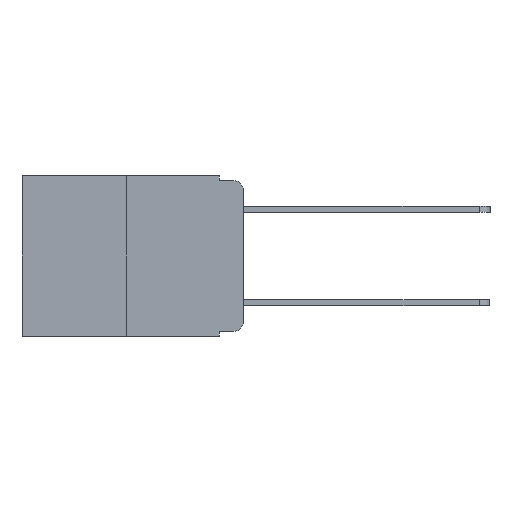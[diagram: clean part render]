
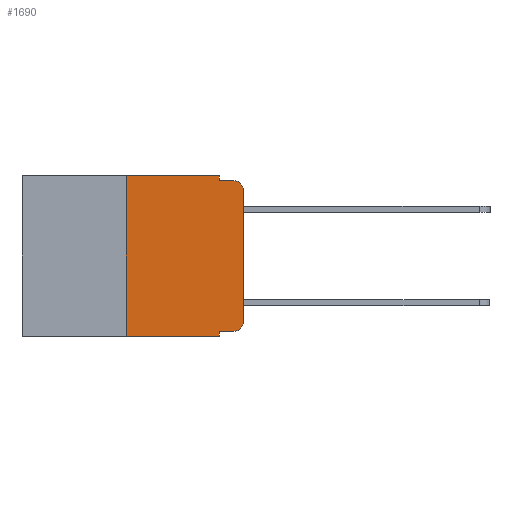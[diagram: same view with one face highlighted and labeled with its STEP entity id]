
A CAD part, left-side view. The second image highlights one B-rep face of the part: STEP entity #1690.
In plain terms, the highlighted planar face has unit normal (-1, 0, 0).
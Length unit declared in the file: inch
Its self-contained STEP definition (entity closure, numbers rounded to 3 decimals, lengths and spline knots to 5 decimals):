
#182 = CARTESIAN_POINT ( 'NONE',  ( 0., 0.051, -0.333 ) ) ;
#215 = VERTEX_POINT ( 'NONE', #10830 ) ;
#274 = VERTEX_POINT ( 'NONE', #9035 ) ;
#319 = AXIS2_PLACEMENT_3D ( 'NONE', #7920, #11043, #8662 ) ;
#332 = DIRECTION ( 'NONE',  ( 0., -1., 0. ) ) ;
#364 = LINE ( 'NONE', #9904, #8075 ) ;
#462 = DIRECTION ( 'NONE',  ( 0., -1., 0. ) ) ;
#549 = AXIS2_PLACEMENT_3D ( 'NONE', #2969, #10202, #4015 ) ;
#583 = ORIENTED_EDGE ( 'NONE', *, *, #964, .F. ) ;
#774 = VERTEX_POINT ( 'NONE', #8952 ) ;
#844 = ORIENTED_EDGE ( 'NONE', *, *, #2609, .F. ) ;
#942 = VECTOR ( 'NONE', #462, 39.37008 ) ;
#964 = EDGE_CURVE ( 'NONE', #8962, #2839, #9199, .T. ) ;
#1352 = VECTOR ( 'NONE', #332, 39.37008 ) ;
#1613 = VERTEX_POINT ( 'NONE', #10440 ) ;
#1676 = ORIENTED_EDGE ( 'NONE', *, *, #7356, .F. ) ;
#1690 = ADVANCED_FACE ( 'NONE', ( #9287 ), #9490, .F. ) ;
#2224 = DIRECTION ( 'NONE',  ( 0., 0., -1. ) ) ;
#2482 = CARTESIAN_POINT ( 'NONE',  ( 0., 0.051, 0. ) ) ;
#2568 = EDGE_CURVE ( 'NONE', #8911, #4649, #6262, .T. ) ;
#2588 = EDGE_CURVE ( 'NONE', #1613, #8962, #10175, .T. ) ;
#2609 = EDGE_CURVE ( 'NONE', #2839, #7768, #3333, .T. ) ;
#2775 = EDGE_LOOP ( 'NONE', ( #2952, #3688, #1676, #844, #583, #6097, #6383, #5727, #5455, #4784 ) ) ;
#2839 = VERTEX_POINT ( 'NONE', #7045 ) ;
#2952 = ORIENTED_EDGE ( 'NONE', *, *, #7534, .T. ) ;
#2969 = CARTESIAN_POINT ( 'NONE',  ( 0., 0.473, 0. ) ) ;
#3315 = DIRECTION ( 'NONE',  ( 0., -1., 0. ) ) ;
#3333 = LINE ( 'NONE', #2482, #9954 ) ;
#3688 = ORIENTED_EDGE ( 'NONE', *, *, #7370, .T. ) ;
#4015 = DIRECTION ( 'NONE',  ( 0., 0., -1. ) ) ;
#4265 = AXIS2_PLACEMENT_3D ( 'NONE', #9642, #4615, #10356 ) ;
#4423 = VERTEX_POINT ( 'NONE', #10189 ) ;
#4615 = DIRECTION ( 'NONE',  ( -1., 0., 0. ) ) ;
#4649 = VERTEX_POINT ( 'NONE', #7971 ) ;
#4715 = DIRECTION ( 'NONE',  ( 0., 0., 1. ) ) ;
#4784 = ORIENTED_EDGE ( 'NONE', *, *, #2568, .T. ) ;
#4799 = CARTESIAN_POINT ( 'NONE',  ( 0., 0.25, 0. ) ) ;
#4866 = LINE ( 'NONE', #10874, #7059 ) ;
#5299 = CARTESIAN_POINT ( 'NONE',  ( 0., 0.473, 0. ) ) ;
#5313 = LINE ( 'NONE', #8994, #9445 ) ;
#5455 = ORIENTED_EDGE ( 'NONE', *, *, #6141, .T. ) ;
#5571 = CARTESIAN_POINT ( 'NONE',  ( 0., 0.051, -0.01 ) ) ;
#5727 = ORIENTED_EDGE ( 'NONE', *, *, #7303, .F. ) ;
#5933 = VECTOR ( 'NONE', #3315, 39.37008 ) ;
#5987 = VECTOR ( 'NONE', #4715, 39.37008 ) ;
#6097 = ORIENTED_EDGE ( 'NONE', *, *, #2588, .F. ) ;
#6141 = EDGE_CURVE ( 'NONE', #774, #8911, #8440, .T. ) ;
#6200 = LINE ( 'NONE', #8152, #942 ) ;
#6262 = CIRCLE ( 'NONE', #319, 0.02 ) ;
#6383 = ORIENTED_EDGE ( 'NONE', *, *, #7399, .T. ) ;
#7045 = CARTESIAN_POINT ( 'NONE',  ( 0., 0.051, 0. ) ) ;
#7059 = VECTOR ( 'NONE', #8056, 39.37008 ) ;
#7303 = EDGE_CURVE ( 'NONE', #774, #274, #4866, .T. ) ;
#7356 = EDGE_CURVE ( 'NONE', #7768, #215, #6200, .T. ) ;
#7370 = EDGE_CURVE ( 'NONE', #4423, #215, #10126, .T. ) ;
#7399 = EDGE_CURVE ( 'NONE', #1613, #274, #5313, .T. ) ;
#7534 = EDGE_CURVE ( 'NONE', #4649, #4423, #364, .T. ) ;
#7768 = VERTEX_POINT ( 'NONE', #5571 ) ;
#7913 = CARTESIAN_POINT ( 'NONE',  ( 0., 0.25, 0. ) ) ;
#7920 = CARTESIAN_POINT ( 'NONE',  ( 0., 0.02, -0.313 ) ) ;
#7971 = CARTESIAN_POINT ( 'NONE',  ( 0., 0., -0.313 ) ) ;
#8056 = DIRECTION ( 'NONE',  ( 0., 0., -1. ) ) ;
#8075 = VECTOR ( 'NONE', #11270, 39.37008 ) ;
#8152 = CARTESIAN_POINT ( 'NONE',  ( 0., 0.051, -0.01 ) ) ;
#8322 = CARTESIAN_POINT ( 'NONE',  ( 0., 0.02, -0.333 ) ) ;
#8440 = LINE ( 'NONE', #182, #5933 ) ;
#8662 = DIRECTION ( 'NONE',  ( 0., 0., -1. ) ) ;
#8911 = VERTEX_POINT ( 'NONE', #8322 ) ;
#8952 = CARTESIAN_POINT ( 'NONE',  ( 0., 0.051, -0.333 ) ) ;
#8962 = VERTEX_POINT ( 'NONE', #4799 ) ;
#8994 = CARTESIAN_POINT ( 'NONE',  ( 0., 0.473, -0.343 ) ) ;
#9035 = CARTESIAN_POINT ( 'NONE',  ( 0., 0.051, -0.343 ) ) ;
#9199 = LINE ( 'NONE', #5299, #1352 ) ;
#9287 = FACE_OUTER_BOUND ( 'NONE', #2775, .T. ) ;
#9445 = VECTOR ( 'NONE', #9709, 39.37008 ) ;
#9490 = PLANE ( 'NONE',  #549 ) ;
#9642 = CARTESIAN_POINT ( 'NONE',  ( 0., 0.02, -0.03 ) ) ;
#9709 = DIRECTION ( 'NONE',  ( 0., -1., 0. ) ) ;
#9904 = CARTESIAN_POINT ( 'NONE',  ( 0., 0., 0. ) ) ;
#9954 = VECTOR ( 'NONE', #2224, 39.37008 ) ;
#10126 = CIRCLE ( 'NONE', #4265, 0.02 ) ;
#10175 = LINE ( 'NONE', #7913, #5987 ) ;
#10189 = CARTESIAN_POINT ( 'NONE',  ( 0., 0., -0.03 ) ) ;
#10202 = DIRECTION ( 'NONE',  ( 1., 0., 0. ) ) ;
#10356 = DIRECTION ( 'NONE',  ( 0., 0., -1. ) ) ;
#10440 = CARTESIAN_POINT ( 'NONE',  ( 0., 0.25, -0.343 ) ) ;
#10830 = CARTESIAN_POINT ( 'NONE',  ( 0., 0.02, -0.01 ) ) ;
#10874 = CARTESIAN_POINT ( 'NONE',  ( 0., 0.051, 0. ) ) ;
#11043 = DIRECTION ( 'NONE',  ( -1., 0., 0. ) ) ;
#11270 = DIRECTION ( 'NONE',  ( 0., 0., 1. ) ) ;
